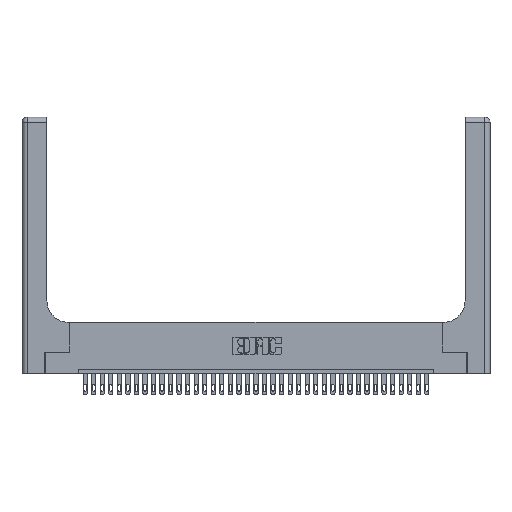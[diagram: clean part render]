
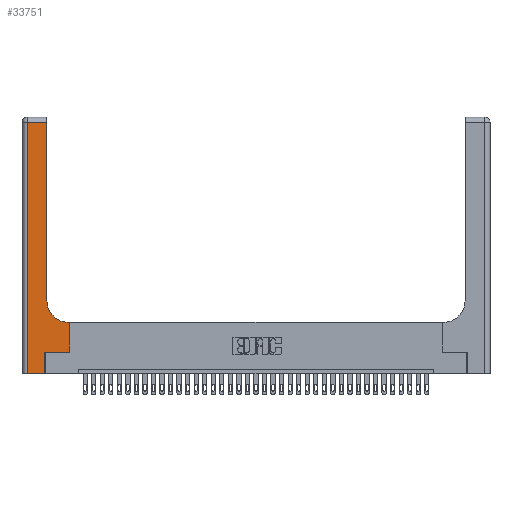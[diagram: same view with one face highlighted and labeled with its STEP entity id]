
A CAD part, top view. The second image highlights one B-rep face of the part: STEP entity #33751.
In plain terms, the highlighted planar face has unit normal (0, 0, 1).
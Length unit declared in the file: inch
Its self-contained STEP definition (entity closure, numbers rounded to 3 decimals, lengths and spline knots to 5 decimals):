
#675 = VECTOR ( 'NONE', #16523, 39.37008 ) ;
#1253 = VERTEX_POINT ( 'NONE', #18215 ) ;
#1536 = EDGE_CURVE ( 'NONE', #23127, #32710, #27244, .T. ) ;
#1635 = CARTESIAN_POINT ( 'NONE',  ( 0.5585, 0.6, 0.37 ) ) ;
#1897 = CARTESIAN_POINT ( 'NONE',  ( 0.269, 0.25, 0.37 ) ) ;
#2208 = VECTOR ( 'NONE', #13161, 39.37008 ) ;
#2334 = VECTOR ( 'NONE', #32724, 39.37008 ) ;
#2363 = DIRECTION ( 'NONE',  ( 0., 0., -1. ) ) ;
#4164 = FACE_OUTER_BOUND ( 'NONE', #4323, .T. ) ;
#4178 = DIRECTION ( 'NONE',  ( -1., 0., 0. ) ) ;
#4323 = EDGE_LOOP ( 'NONE', ( #12181, #27021, #31408, #28081, #28528, #34348, #34384, #26232, #17634 ) ) ;
#5474 = CARTESIAN_POINT ( 'NONE',  ( 0.5415, 0.85, 0.37 ) ) ;
#6222 = EDGE_CURVE ( 'NONE', #1253, #22694, #35353, .T. ) ;
#6672 = VECTOR ( 'NONE', #11994, 39.37008 ) ;
#6833 = CARTESIAN_POINT ( 'NONE',  ( 0., 3., 0.37 ) ) ;
#8498 = CARTESIAN_POINT ( 'NONE',  ( 0.5415, 0.6, 0.37 ) ) ;
#8796 = AXIS2_PLACEMENT_3D ( 'NONE', #5474, #2363, #35964 ) ;
#9597 = DIRECTION ( 'NONE',  ( 0., 0., -1. ) ) ;
#9893 = VERTEX_POINT ( 'NONE', #11940 ) ;
#10342 = DIRECTION ( 'NONE',  ( 0., 1., 0. ) ) ;
#10766 = CARTESIAN_POINT ( 'NONE',  ( 0., 2.94, 0.37 ) ) ;
#11361 = VECTOR ( 'NONE', #10342, 39.37008 ) ;
#11860 = CARTESIAN_POINT ( 'NONE',  ( 0.2915, 0.6, 0.37 ) ) ;
#11940 = CARTESIAN_POINT ( 'NONE',  ( 0.06, 2.94, 0.37 ) ) ;
#11994 = DIRECTION ( 'NONE',  ( -1., 0., 0. ) ) ;
#12181 = ORIENTED_EDGE ( 'NONE', *, *, #6222, .T. ) ;
#12497 = CARTESIAN_POINT ( 'NONE',  ( 0.2915, 3., 0.37 ) ) ;
#12732 = CARTESIAN_POINT ( 'NONE',  ( 0.269, 0.25, 0.37 ) ) ;
#13161 = DIRECTION ( 'NONE',  ( 1., 0., 0. ) ) ;
#14036 = LINE ( 'NONE', #11860, #6672 ) ;
#14313 = VECTOR ( 'NONE', #21162, 39.37008 ) ;
#14710 = VERTEX_POINT ( 'NONE', #31967 ) ;
#14862 = PLANE ( 'NONE',  #22110 ) ;
#15946 = DIRECTION ( 'NONE',  ( 0., 1., 0. ) ) ;
#16523 = DIRECTION ( 'NONE',  ( 1., 0., 0. ) ) ;
#16734 = EDGE_CURVE ( 'NONE', #9893, #14710, #18418, .T. ) ;
#17217 = CIRCLE ( 'NONE', #8796, 0.25 ) ;
#17634 = ORIENTED_EDGE ( 'NONE', *, *, #21352, .T. ) ;
#18215 = CARTESIAN_POINT ( 'NONE',  ( 0.2915, 0.85, 0.37 ) ) ;
#18418 = LINE ( 'NONE', #32402, #2334 ) ;
#18567 = LINE ( 'NONE', #33334, #675 ) ;
#18998 = EDGE_CURVE ( 'NONE', #32710, #29855, #28220, .T. ) ;
#21162 = DIRECTION ( 'NONE',  ( 0., 1., 0. ) ) ;
#21352 = EDGE_CURVE ( 'NONE', #30714, #1253, #17217, .T. ) ;
#21385 = CARTESIAN_POINT ( 'NONE',  ( 0.2915, 2.94, 0.37 ) ) ;
#22110 = AXIS2_PLACEMENT_3D ( 'NONE', #6833, #9597, #4178 ) ;
#22694 = VERTEX_POINT ( 'NONE', #21385 ) ;
#22822 = CARTESIAN_POINT ( 'NONE',  ( 0.269, 0., 0.37 ) ) ;
#23127 = VERTEX_POINT ( 'NONE', #22822 ) ;
#23649 = EDGE_CURVE ( 'NONE', #14710, #23127, #18567, .T. ) ;
#25825 = EDGE_CURVE ( 'NONE', #22694, #9893, #35441, .T. ) ;
#26232 = ORIENTED_EDGE ( 'NONE', *, *, #29549, .T. ) ;
#27021 = ORIENTED_EDGE ( 'NONE', *, *, #25825, .T. ) ;
#27244 = LINE ( 'NONE', #29808, #33764 ) ;
#28081 = ORIENTED_EDGE ( 'NONE', *, *, #23649, .T. ) ;
#28220 = LINE ( 'NONE', #1897, #2208 ) ;
#28528 = ORIENTED_EDGE ( 'NONE', *, *, #1536, .T. ) ;
#29318 = EDGE_CURVE ( 'NONE', #29855, #30971, #35487, .T. ) ;
#29549 = EDGE_CURVE ( 'NONE', #30971, #30714, #14036, .T. ) ;
#29808 = CARTESIAN_POINT ( 'NONE',  ( 0.269, 0., 0.37 ) ) ;
#29855 = VERTEX_POINT ( 'NONE', #35921 ) ;
#30383 = DIRECTION ( 'NONE',  ( -1., 0., 0. ) ) ;
#30714 = VERTEX_POINT ( 'NONE', #8498 ) ;
#30971 = VERTEX_POINT ( 'NONE', #1635 ) ;
#31408 = ORIENTED_EDGE ( 'NONE', *, *, #16734, .T. ) ;
#31472 = VECTOR ( 'NONE', #30383, 39.37008 ) ;
#31967 = CARTESIAN_POINT ( 'NONE',  ( 0.06, 0., 0.37 ) ) ;
#32402 = CARTESIAN_POINT ( 'NONE',  ( 0.06, 3., 0.37 ) ) ;
#32710 = VERTEX_POINT ( 'NONE', #12732 ) ;
#32724 = DIRECTION ( 'NONE',  ( 0., -1., 0. ) ) ;
#33334 = CARTESIAN_POINT ( 'NONE',  ( 0., 0., 0.37 ) ) ;
#33751 = ADVANCED_FACE ( 'NONE', ( #4164 ), #14862, .F. ) ;
#33764 = VECTOR ( 'NONE', #15946, 39.37008 ) ;
#34348 = ORIENTED_EDGE ( 'NONE', *, *, #18998, .T. ) ;
#34384 = ORIENTED_EDGE ( 'NONE', *, *, #29318, .T. ) ;
#35353 = LINE ( 'NONE', #12497, #14313 ) ;
#35441 = LINE ( 'NONE', #10766, #31472 ) ;
#35487 = LINE ( 'NONE', #35618, #11361 ) ;
#35618 = CARTESIAN_POINT ( 'NONE',  ( 0.5585, 0.25, 0.37 ) ) ;
#35921 = CARTESIAN_POINT ( 'NONE',  ( 0.5585, 0.25, 0.37 ) ) ;
#35964 = DIRECTION ( 'NONE',  ( 1., 0., 0. ) ) ;
